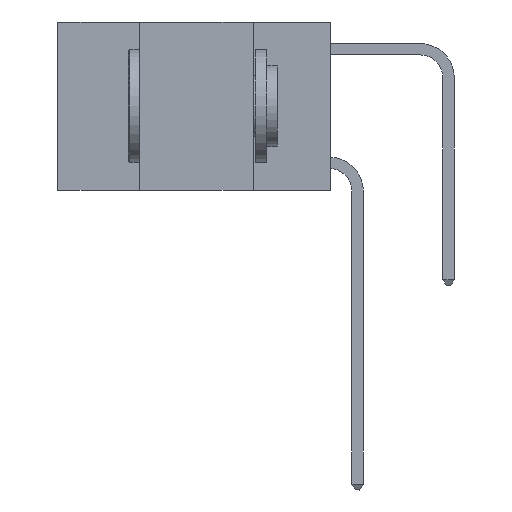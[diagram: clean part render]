
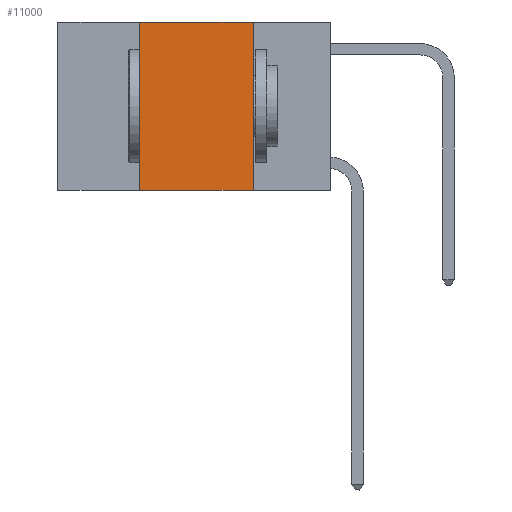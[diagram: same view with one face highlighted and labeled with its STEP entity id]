
A CAD part, left-side view. The second image highlights one B-rep face of the part: STEP entity #11000.
In plain terms, the highlighted planar face has unit normal (-1, 0, 0).
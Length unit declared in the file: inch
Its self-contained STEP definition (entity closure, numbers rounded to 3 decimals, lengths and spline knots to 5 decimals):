
#387 = EDGE_LOOP ( 'NONE', ( #8344, #20622, #12555, #22800 ) ) ;
#690 = VERTEX_POINT ( 'NONE', #20225 ) ;
#888 = LINE ( 'NONE', #31452, #5347 ) ;
#4860 = LINE ( 'NONE', #24700, #15965 ) ;
#4890 = PLANE ( 'NONE',  #23455 ) ;
#5347 = VECTOR ( 'NONE', #16187, 39.37008 ) ;
#8058 = VECTOR ( 'NONE', #27121, 39.37008 ) ;
#8344 = ORIENTED_EDGE ( 'NONE', *, *, #20476, .F. ) ;
#11000 = ADVANCED_FACE ( 'NONE', ( #19379 ), #4890, .F. ) ;
#12555 = ORIENTED_EDGE ( 'NONE', *, *, #27466, .F. ) ;
#13057 = VERTEX_POINT ( 'NONE', #22813 ) ;
#14255 = CARTESIAN_POINT ( 'NONE',  ( 0., 0.6, 0. ) ) ;
#14745 = DIRECTION ( 'NONE',  ( 0., 0., -1. ) ) ;
#15965 = VECTOR ( 'NONE', #27959, 39.37008 ) ;
#16187 = DIRECTION ( 'NONE',  ( 0., 0., 1. ) ) ;
#18716 = EDGE_CURVE ( 'NONE', #13057, #20526, #31265, .T. ) ;
#19075 = EDGE_CURVE ( 'NONE', #22417, #690, #4860, .T. ) ;
#19379 = FACE_OUTER_BOUND ( 'NONE', #387, .T. ) ;
#20219 = CARTESIAN_POINT ( 'NONE',  ( 0., 0.42, -0.37 ) ) ;
#20225 = CARTESIAN_POINT ( 'NONE',  ( 0., 0.17, -0.37 ) ) ;
#20476 = EDGE_CURVE ( 'NONE', #20526, #690, #20681, .T. ) ;
#20526 = VERTEX_POINT ( 'NONE', #25686 ) ;
#20622 = ORIENTED_EDGE ( 'NONE', *, *, #18716, .F. ) ;
#20681 = LINE ( 'NONE', #30825, #23910 ) ;
#22417 = VERTEX_POINT ( 'NONE', #20219 ) ;
#22722 = CARTESIAN_POINT ( 'NONE',  ( 0., 0.6, 0. ) ) ;
#22800 = ORIENTED_EDGE ( 'NONE', *, *, #19075, .T. ) ;
#22813 = CARTESIAN_POINT ( 'NONE',  ( 0., 0.42, 0. ) ) ;
#23455 = AXIS2_PLACEMENT_3D ( 'NONE', #22722, #30472, #33023 ) ;
#23910 = VECTOR ( 'NONE', #14745, 39.37008 ) ;
#24700 = CARTESIAN_POINT ( 'NONE',  ( 0., 0.6, -0.37 ) ) ;
#25686 = CARTESIAN_POINT ( 'NONE',  ( 0., 0.17, 0. ) ) ;
#27121 = DIRECTION ( 'NONE',  ( 0., -1., 0. ) ) ;
#27466 = EDGE_CURVE ( 'NONE', #22417, #13057, #888, .T. ) ;
#27959 = DIRECTION ( 'NONE',  ( 0., -1., 0. ) ) ;
#30472 = DIRECTION ( 'NONE',  ( 1., 0., 0. ) ) ;
#30825 = CARTESIAN_POINT ( 'NONE',  ( 0., 0.17, 0. ) ) ;
#31265 = LINE ( 'NONE', #14255, #8058 ) ;
#31452 = CARTESIAN_POINT ( 'NONE',  ( 0., 0.42, 0. ) ) ;
#33023 = DIRECTION ( 'NONE',  ( 0., 0., -1. ) ) ;
